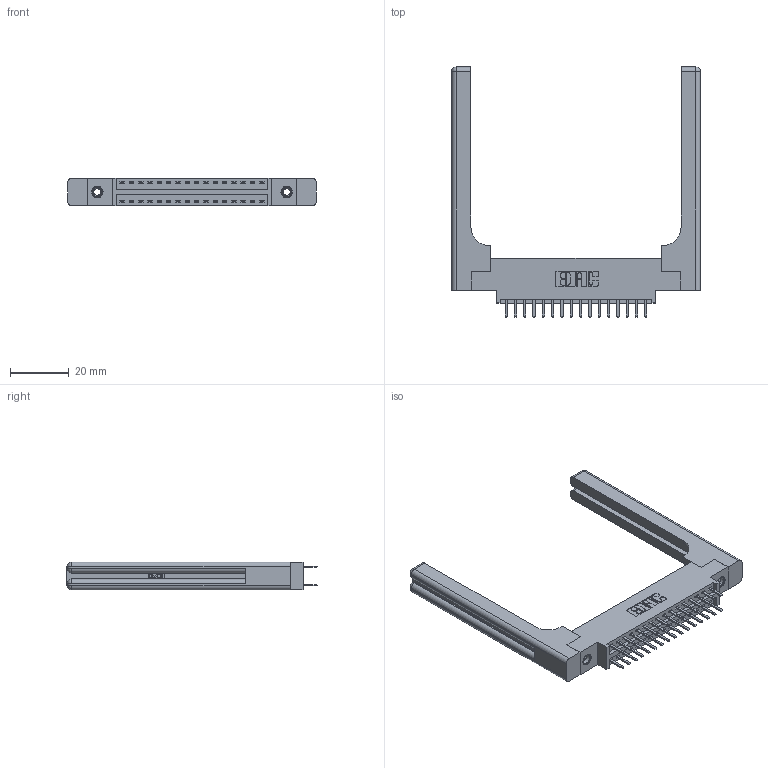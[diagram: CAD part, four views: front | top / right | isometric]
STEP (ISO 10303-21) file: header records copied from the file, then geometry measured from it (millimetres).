
FILE_DESCRIPTION (( 'STEP AP203' ), '1' );
FILE_NAME ('346-032-520-858.STEP', '2022-05-19T17:34:00', ( '' ), ( '' ), 'SwSTEP 2.0', 'SolidWorks 2020', '' );
FILE_SCHEMA (( 'CONFIG_CONTROL_DESIGN' ));
Length unit declared in the file: inch
Products named in the file (5): 346-220-058_345-220-058; 345-292-001_345-293-120; 346-032-520-858; 345-250-001_345-250-001-102; 346 Part_0.170 Offset - 0.156 Dia-TH
Assembly tree (37 placements, depth 2):
  346-032-520-858
    346 Part_0.170 Offset - 0.156 Dia-TH
    345-292-001_345-293-120  x32
    345-250-001_345-250-001-102  x2
    346-220-058_345-220-058  x2
Bounding box: 84.86 x 85.29 x 9.4 mm (x, y, z)
Volume: 15380.6 mm3; surface area: 15585.6 mm2
Topology: 37 solids, 37 shells, 2188 faces, 6259 edges, 4066 vertices
Faces by surface type: plane 1426, cylinder 702, bspline 36, cone 12, sphere 8, torus 4
Entity records: 19786 total; most frequent: CARTESIAN_POINT 4323, ORIENTED_EDGE 3040, DIRECTION 2780, EDGE_CURVE 1520, LINE 1228, VECTOR 1228, VERTEX_POINT 1002, AXIS2_PLACEMENT_3D 776
